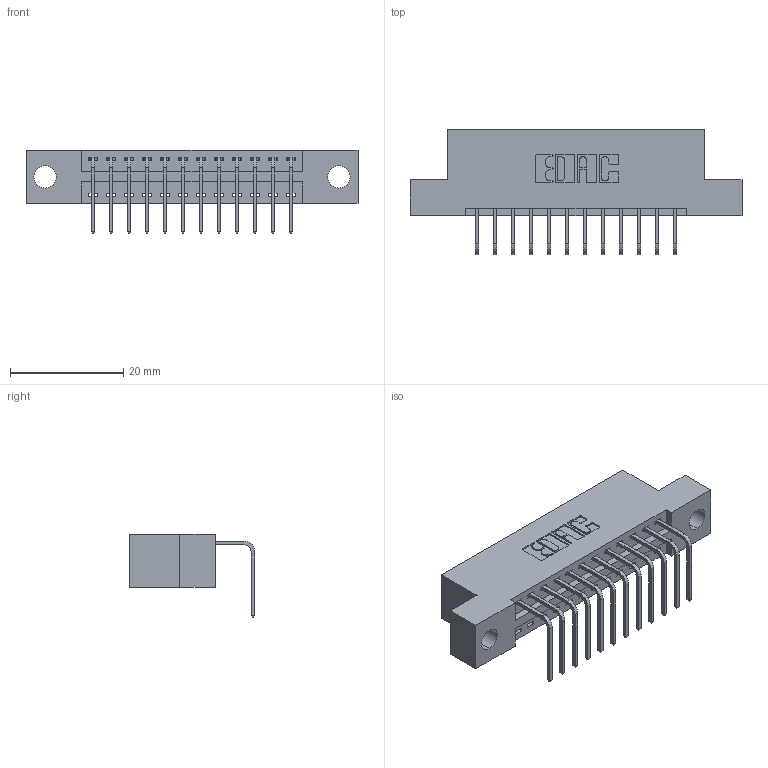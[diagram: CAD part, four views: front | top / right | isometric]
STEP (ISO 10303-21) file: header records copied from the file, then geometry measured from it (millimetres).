
FILE_DESCRIPTION (( 'STEP AP203' ), '1' );
FILE_NAME ('396-012-558-104.STEP', '2018-08-31T07:04:02', ( '' ), ( '' ), 'SwSTEP 2.0', 'SolidWorks 2016', '' );
FILE_SCHEMA (( 'CONFIG_CONTROL_DESIGN' ));
Length unit declared in the file: inch
Products named in the file (3): 346 Part_Flush Mounting Lugs - 0.156 Dia-TH; 345-292-001_558 Tail - 2; 396-012-558-104
Assembly tree (13 placements, depth 2):
  396-012-558-104
    346 Part_Flush Mounting Lugs - 0.156 Dia-TH
    345-292-001_558 Tail - 2  x12
Bounding box: 58.67 x 22.16 x 14.73 mm (x, y, z)
Volume: 5361.8 mm3; surface area: 6421.4 mm2
Topology: 13 solids, 13 shells, 842 faces, 2513 edges, 1658 vertices
Faces by surface type: plane 580, cylinder 262
Entity records: 11573 total; most frequent: CARTESIAN_POINT 2000, ORIENTED_EDGE 1946, DIRECTION 1801, EDGE_CURVE 973, LINE 793, VECTOR 793, VERTEX_POINT 646, AXIS2_PLACEMENT_3D 504
